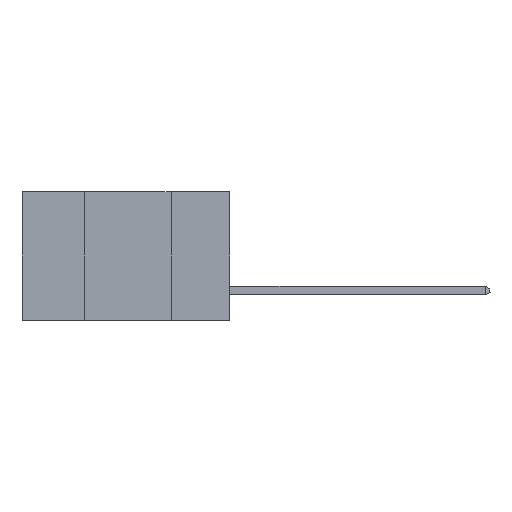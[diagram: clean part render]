
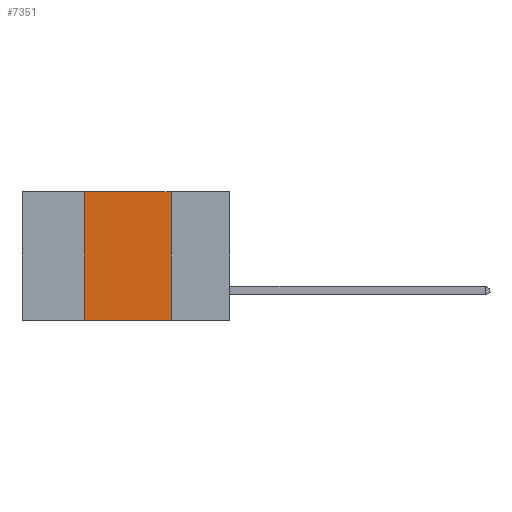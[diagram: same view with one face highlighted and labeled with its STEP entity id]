
A CAD part, left-side view. The second image highlights one B-rep face of the part: STEP entity #7351.
In plain terms, the highlighted planar face has unit normal (-1, 0, 0).
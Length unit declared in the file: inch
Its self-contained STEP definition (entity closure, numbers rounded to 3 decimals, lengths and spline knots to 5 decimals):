
#513 = CARTESIAN_POINT ( 'NONE',  ( 0., 0.17, 0. ) ) ;
#548 = DIRECTION ( 'NONE',  ( 0., 0., -1. ) ) ;
#1011 = EDGE_CURVE ( 'NONE', #22390, #5451, #27555, .T. ) ;
#2035 = EDGE_CURVE ( 'NONE', #5451, #27808, #8262, .T. ) ;
#3918 = ORIENTED_EDGE ( 'NONE', *, *, #11831, .F. ) ;
#4057 = VECTOR ( 'NONE', #8298, 39.37008 ) ;
#4309 = FACE_OUTER_BOUND ( 'NONE', #5158, .T. ) ;
#4814 = LINE ( 'NONE', #25479, #27059 ) ;
#5158 = EDGE_LOOP ( 'NONE', ( #25157, #7226, #3918, #16446 ) ) ;
#5451 = VERTEX_POINT ( 'NONE', #513 ) ;
#7226 = ORIENTED_EDGE ( 'NONE', *, *, #1011, .F. ) ;
#7351 = ADVANCED_FACE ( 'NONE', ( #4309 ), #7432, .F. ) ;
#7432 = PLANE ( 'NONE',  #9325 ) ;
#7545 = CARTESIAN_POINT ( 'NONE',  ( 0., 0.42, -0.37 ) ) ;
#8262 = LINE ( 'NONE', #22665, #4057 ) ;
#8298 = DIRECTION ( 'NONE',  ( 0., 0., -1. ) ) ;
#9325 = AXIS2_PLACEMENT_3D ( 'NONE', #29917, #15059, #548 ) ;
#9901 = VECTOR ( 'NONE', #19964, 39.37008 ) ;
#10849 = VECTOR ( 'NONE', #21224, 39.37008 ) ;
#11831 = EDGE_CURVE ( 'NONE', #15157, #22390, #4814, .T. ) ;
#15059 = DIRECTION ( 'NONE',  ( 1., 0., 0. ) ) ;
#15157 = VERTEX_POINT ( 'NONE', #7545 ) ;
#15527 = EDGE_CURVE ( 'NONE', #15157, #27808, #28083, .T. ) ;
#16446 = ORIENTED_EDGE ( 'NONE', *, *, #15527, .T. ) ;
#16644 = CARTESIAN_POINT ( 'NONE',  ( 0., 0.6, -0.37 ) ) ;
#19282 = CARTESIAN_POINT ( 'NONE',  ( 0., 0.42, 0. ) ) ;
#19964 = DIRECTION ( 'NONE',  ( 0., -1., 0. ) ) ;
#20933 = CARTESIAN_POINT ( 'NONE',  ( 0., 0.17, -0.37 ) ) ;
#21224 = DIRECTION ( 'NONE',  ( 0., -1., 0. ) ) ;
#22390 = VERTEX_POINT ( 'NONE', #19282 ) ;
#22665 = CARTESIAN_POINT ( 'NONE',  ( 0., 0.17, 0. ) ) ;
#25157 = ORIENTED_EDGE ( 'NONE', *, *, #2035, .F. ) ;
#25479 = CARTESIAN_POINT ( 'NONE',  ( 0., 0.42, 0. ) ) ;
#27059 = VECTOR ( 'NONE', #27834, 39.37008 ) ;
#27555 = LINE ( 'NONE', #29927, #9901 ) ;
#27808 = VERTEX_POINT ( 'NONE', #20933 ) ;
#27834 = DIRECTION ( 'NONE',  ( 0., 0., 1. ) ) ;
#28083 = LINE ( 'NONE', #16644, #10849 ) ;
#29917 = CARTESIAN_POINT ( 'NONE',  ( 0., 0.6, 0. ) ) ;
#29927 = CARTESIAN_POINT ( 'NONE',  ( 0., 0.6, 0. ) ) ;
